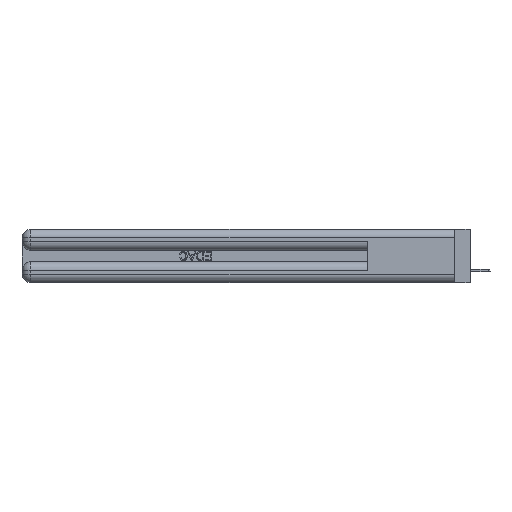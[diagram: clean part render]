
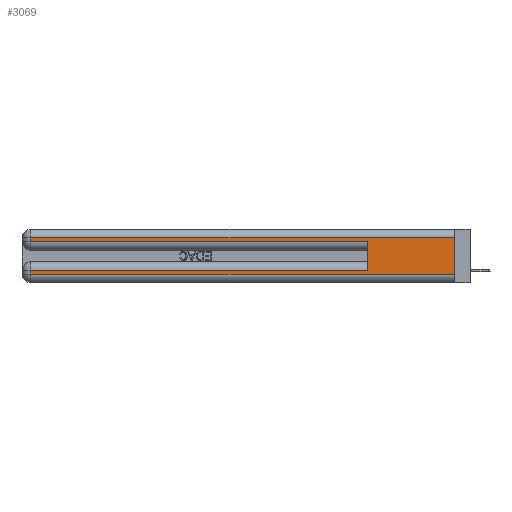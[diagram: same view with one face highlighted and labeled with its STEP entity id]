
A CAD part, left-side view. The second image highlights one B-rep face of the part: STEP entity #3069.
In plain terms, the highlighted planar face has unit normal (-1, 0, 0).
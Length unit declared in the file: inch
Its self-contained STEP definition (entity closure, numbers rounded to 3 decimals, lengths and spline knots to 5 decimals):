
#292 = DIRECTION ( 'NONE',  ( 0., 1., 0. ) ) ;
#721 = CARTESIAN_POINT ( 'NONE',  ( 0., 0., 0.06 ) ) ;
#1865 = ORIENTED_EDGE ( 'NONE', *, *, #33917, .T. ) ;
#2503 = DIRECTION ( 'NONE',  ( 0., 0., -1. ) ) ;
#3069 = ADVANCED_FACE ( 'NONE', ( #15001 ), #44057, .F. ) ;
#3198 = VECTOR ( 'NONE', #292, 39.37008 ) ;
#3517 = VECTOR ( 'NONE', #18800, 39.37008 ) ;
#3585 = DIRECTION ( 'NONE',  ( 0., 0., -1. ) ) ;
#4095 = CARTESIAN_POINT ( 'NONE',  ( 0., 0., 0.085 ) ) ;
#4658 = CARTESIAN_POINT ( 'NONE',  ( 0., 2.94, 0.37 ) ) ;
#6320 = DIRECTION ( 'NONE',  ( 1., 0., 0. ) ) ;
#7327 = CARTESIAN_POINT ( 'NONE',  ( 0., 0., 0.31 ) ) ;
#7330 = CARTESIAN_POINT ( 'NONE',  ( 0., 2.94, 0.31 ) ) ;
#9588 = LINE ( 'NONE', #39439, #33082 ) ;
#10118 = VERTEX_POINT ( 'NONE', #52978 ) ;
#11839 = EDGE_LOOP ( 'NONE', ( #21682, #1865, #37533, #24356, #53490, #46516, #15664, #47024 ) ) ;
#12233 = LINE ( 'NONE', #4095, #3198 ) ;
#13094 = CARTESIAN_POINT ( 'NONE',  ( 0., 0., 0.285 ) ) ;
#13533 = CARTESIAN_POINT ( 'NONE',  ( 0., 0.6, 0.085 ) ) ;
#15001 = FACE_OUTER_BOUND ( 'NONE', #11839, .T. ) ;
#15082 = CARTESIAN_POINT ( 'NONE',  ( 0., 0., 0.06 ) ) ;
#15446 = EDGE_CURVE ( 'NONE', #10118, #35512, #51758, .T. ) ;
#15664 = ORIENTED_EDGE ( 'NONE', *, *, #20671, .T. ) ;
#17330 = CARTESIAN_POINT ( 'NONE',  ( 0., 0., 0.31 ) ) ;
#18800 = DIRECTION ( 'NONE',  ( 0., 0., -1. ) ) ;
#20671 = EDGE_CURVE ( 'NONE', #33282, #10118, #41845, .T. ) ;
#20893 = CARTESIAN_POINT ( 'NONE',  ( 0., 0.6, 0.145 ) ) ;
#21682 = ORIENTED_EDGE ( 'NONE', *, *, #23751, .F. ) ;
#22965 = LINE ( 'NONE', #17330, #43070 ) ;
#23751 = EDGE_CURVE ( 'NONE', #34723, #35512, #39150, .T. ) ;
#23952 = DIRECTION ( 'NONE',  ( 0., 0., -1. ) ) ;
#24356 = ORIENTED_EDGE ( 'NONE', *, *, #45618, .T. ) ;
#27659 = CARTESIAN_POINT ( 'NONE',  ( 0., 2.94, 0.085 ) ) ;
#29978 = AXIS2_PLACEMENT_3D ( 'NONE', #44318, #6320, #23952 ) ;
#30351 = VERTEX_POINT ( 'NONE', #7330 ) ;
#30464 = EDGE_CURVE ( 'NONE', #43350, #43151, #37983, .T. ) ;
#32541 = VECTOR ( 'NONE', #45866, 39.37008 ) ;
#33082 = VECTOR ( 'NONE', #2503, 39.37008 ) ;
#33282 = VERTEX_POINT ( 'NONE', #27659 ) ;
#33639 = DIRECTION ( 'NONE',  ( 0., 1., 0. ) ) ;
#33917 = EDGE_CURVE ( 'NONE', #34723, #30351, #22965, .T. ) ;
#34723 = VERTEX_POINT ( 'NONE', #7327 ) ;
#35512 = VERTEX_POINT ( 'NONE', #721 ) ;
#35891 = VECTOR ( 'NONE', #43327, 39.37008 ) ;
#37533 = ORIENTED_EDGE ( 'NONE', *, *, #39677, .T. ) ;
#37815 = LINE ( 'NONE', #13094, #42062 ) ;
#37983 = LINE ( 'NONE', #20893, #32541 ) ;
#39150 = LINE ( 'NONE', #51122, #3517 ) ;
#39439 = CARTESIAN_POINT ( 'NONE',  ( 0., 2.94, 0.37 ) ) ;
#39677 = EDGE_CURVE ( 'NONE', #30351, #43998, #9588, .T. ) ;
#41845 = LINE ( 'NONE', #4658, #51779 ) ;
#42062 = VECTOR ( 'NONE', #49239, 39.37008 ) ;
#43070 = VECTOR ( 'NONE', #33639, 39.37008 ) ;
#43151 = VERTEX_POINT ( 'NONE', #52414 ) ;
#43327 = DIRECTION ( 'NONE',  ( 0., -1., 0. ) ) ;
#43350 = VERTEX_POINT ( 'NONE', #13533 ) ;
#43998 = VERTEX_POINT ( 'NONE', #44931 ) ;
#44057 = PLANE ( 'NONE',  #29978 ) ;
#44318 = CARTESIAN_POINT ( 'NONE',  ( 0., 0., 0.37 ) ) ;
#44931 = CARTESIAN_POINT ( 'NONE',  ( 0., 2.94, 0.285 ) ) ;
#45618 = EDGE_CURVE ( 'NONE', #43998, #43151, #37815, .T. ) ;
#45866 = DIRECTION ( 'NONE',  ( 0., 0., 1. ) ) ;
#46516 = ORIENTED_EDGE ( 'NONE', *, *, #47280, .T. ) ;
#47024 = ORIENTED_EDGE ( 'NONE', *, *, #15446, .T. ) ;
#47280 = EDGE_CURVE ( 'NONE', #43350, #33282, #12233, .T. ) ;
#49239 = DIRECTION ( 'NONE',  ( 0., -1., 0. ) ) ;
#51122 = CARTESIAN_POINT ( 'NONE',  ( 0., 0., 0.37 ) ) ;
#51758 = LINE ( 'NONE', #15082, #35891 ) ;
#51779 = VECTOR ( 'NONE', #3585, 39.37008 ) ;
#52414 = CARTESIAN_POINT ( 'NONE',  ( 0., 0.6, 0.285 ) ) ;
#52978 = CARTESIAN_POINT ( 'NONE',  ( 0., 2.94, 0.06 ) ) ;
#53490 = ORIENTED_EDGE ( 'NONE', *, *, #30464, .F. ) ;
